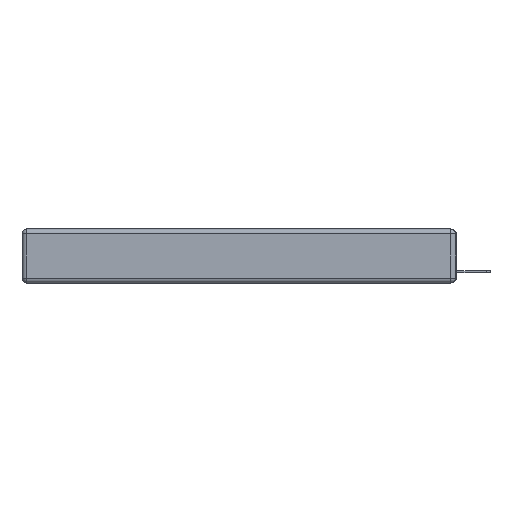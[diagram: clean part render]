
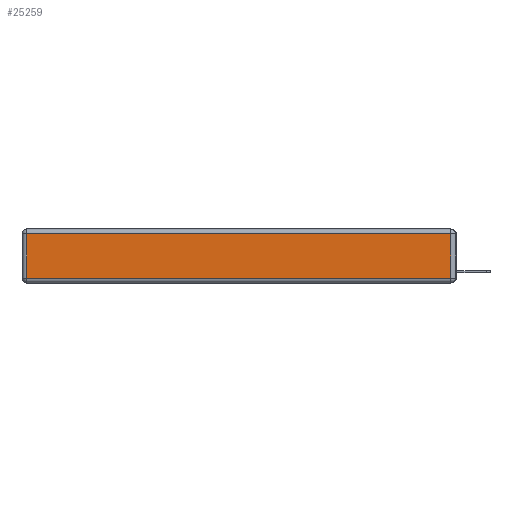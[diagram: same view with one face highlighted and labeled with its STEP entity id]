
A CAD part, left-side view. The second image highlights one B-rep face of the part: STEP entity #25259.
In plain terms, the highlighted planar face has unit normal (-1, 0, 0).
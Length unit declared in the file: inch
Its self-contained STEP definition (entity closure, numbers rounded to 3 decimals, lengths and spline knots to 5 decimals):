
#457 = VECTOR ( 'NONE', #8773, 39.37008 ) ;
#749 = LINE ( 'NONE', #20696, #5900 ) ;
#817 = ORIENTED_EDGE ( 'NONE', *, *, #5783, .T. ) ;
#2249 = VECTOR ( 'NONE', #16284, 39.37008 ) ;
#3159 = CARTESIAN_POINT ( 'NONE',  ( 0., 0.03, -0.03 ) ) ;
#3588 = LINE ( 'NONE', #14145, #2249 ) ;
#5783 = EDGE_CURVE ( 'NONE', #6131, #26974, #749, .T. ) ;
#5900 = VECTOR ( 'NONE', #16585, 39.37008 ) ;
#6131 = VERTEX_POINT ( 'NONE', #6856 ) ;
#6178 = LINE ( 'NONE', #26143, #457 ) ;
#6856 = CARTESIAN_POINT ( 'NONE',  ( 0., 2.72, -0.313 ) ) ;
#8447 = DIRECTION ( 'NONE',  ( 0., 0., 1. ) ) ;
#8724 = CARTESIAN_POINT ( 'NONE',  ( 0., 2.75, -0.03 ) ) ;
#8773 = DIRECTION ( 'NONE',  ( 0., 0., -1. ) ) ;
#10043 = ORIENTED_EDGE ( 'NONE', *, *, #11154, .T. ) ;
#10719 = CARTESIAN_POINT ( 'NONE',  ( 0., 0., -0.343 ) ) ;
#11154 = EDGE_CURVE ( 'NONE', #26974, #16248, #3588, .T. ) ;
#11944 = FACE_OUTER_BOUND ( 'NONE', #20298, .T. ) ;
#12944 = DIRECTION ( 'NONE',  ( -1., 0., 0. ) ) ;
#13049 = PLANE ( 'NONE',  #13787 ) ;
#13198 = CARTESIAN_POINT ( 'NONE',  ( 0., 0.03, -0.313 ) ) ;
#13297 = DIRECTION ( 'NONE',  ( 0., 1., 0. ) ) ;
#13787 = AXIS2_PLACEMENT_3D ( 'NONE', #10719, #12944, #8447 ) ;
#14145 = CARTESIAN_POINT ( 'NONE',  ( 0., 0.03, -0.343 ) ) ;
#15374 = VECTOR ( 'NONE', #13297, 39.37008 ) ;
#16248 = VERTEX_POINT ( 'NONE', #3159 ) ;
#16284 = DIRECTION ( 'NONE',  ( 0., 0., 1. ) ) ;
#16585 = DIRECTION ( 'NONE',  ( 0., -1., 0. ) ) ;
#17168 = VERTEX_POINT ( 'NONE', #19388 ) ;
#19388 = CARTESIAN_POINT ( 'NONE',  ( 0., 2.72, -0.03 ) ) ;
#20298 = EDGE_LOOP ( 'NONE', ( #817, #10043, #24854, #25945 ) ) ;
#20364 = LINE ( 'NONE', #8724, #15374 ) ;
#20696 = CARTESIAN_POINT ( 'NONE',  ( 0., 0., -0.313 ) ) ;
#21319 = EDGE_CURVE ( 'NONE', #16248, #17168, #20364, .T. ) ;
#24854 = ORIENTED_EDGE ( 'NONE', *, *, #21319, .T. ) ;
#25259 = ADVANCED_FACE ( 'NONE', ( #11944 ), #13049, .T. ) ;
#25845 = EDGE_CURVE ( 'NONE', #17168, #6131, #6178, .T. ) ;
#25945 = ORIENTED_EDGE ( 'NONE', *, *, #25845, .T. ) ;
#26143 = CARTESIAN_POINT ( 'NONE',  ( 0., 2.72, -0.343 ) ) ;
#26974 = VERTEX_POINT ( 'NONE', #13198 ) ;
